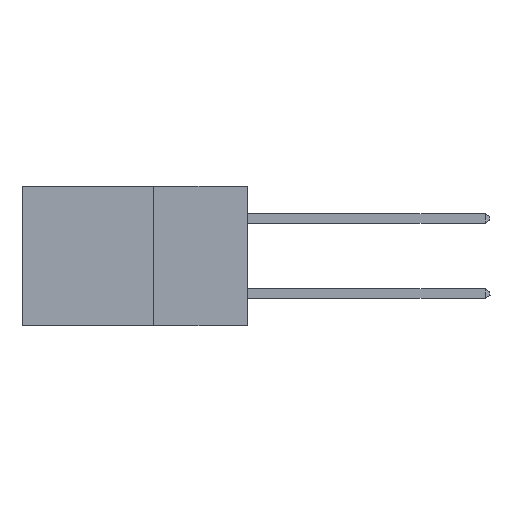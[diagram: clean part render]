
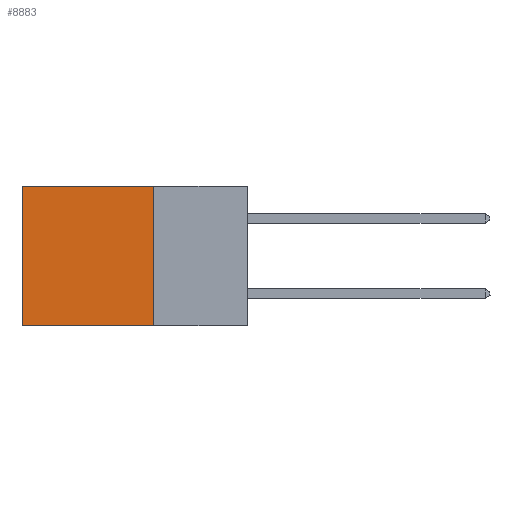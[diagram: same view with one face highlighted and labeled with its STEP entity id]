
A CAD part, left-side view. The second image highlights one B-rep face of the part: STEP entity #8883.
In plain terms, the highlighted planar face has unit normal (-1, 0, 0).
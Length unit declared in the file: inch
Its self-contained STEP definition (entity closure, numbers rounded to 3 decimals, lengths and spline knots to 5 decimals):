
#1209 = DIRECTION ( 'NONE',  ( 0., 0., -1. ) ) ;
#1258 = CARTESIAN_POINT ( 'NONE',  ( 0.298, 0.6, 0. ) ) ;
#1451 = CARTESIAN_POINT ( 'NONE',  ( 0.298, 0.6, 0. ) ) ;
#2287 = AXIS2_PLACEMENT_3D ( 'NONE', #20778, #7983, #25866 ) ;
#2558 = DIRECTION ( 'NONE',  ( 0., 1., 0. ) ) ;
#2759 = EDGE_CURVE ( 'NONE', #10760, #15663, #7163, .T. ) ;
#2866 = PLANE ( 'NONE',  #2287 ) ;
#3177 = EDGE_CURVE ( 'NONE', #23032, #15663, #19971, .T. ) ;
#6310 = VECTOR ( 'NONE', #15525, 39.37008 ) ;
#6875 = EDGE_CURVE ( 'NONE', #24932, #23032, #23200, .T. ) ;
#7163 = LINE ( 'NONE', #24477, #32726 ) ;
#7983 = DIRECTION ( 'NONE',  ( 1., 0., 0. ) ) ;
#8221 = EDGE_CURVE ( 'NONE', #24932, #10760, #19935, .T. ) ;
#8757 = VECTOR ( 'NONE', #2558, 39.37008 ) ;
#8883 = ADVANCED_FACE ( 'NONE', ( #32237 ), #2866, .F. ) ;
#10760 = VERTEX_POINT ( 'NONE', #13992 ) ;
#13992 = CARTESIAN_POINT ( 'NONE',  ( 0.298, 0.25, -0.37 ) ) ;
#15293 = CARTESIAN_POINT ( 'NONE',  ( 0.298, 0.25, 0. ) ) ;
#15525 = DIRECTION ( 'NONE',  ( 0., 0., -1. ) ) ;
#15663 = VERTEX_POINT ( 'NONE', #16317 ) ;
#16317 = CARTESIAN_POINT ( 'NONE',  ( 0.298, 0.6, -0.37 ) ) ;
#18099 = ORIENTED_EDGE ( 'NONE', *, *, #6875, .T. ) ;
#19935 = LINE ( 'NONE', #25678, #6310 ) ;
#19971 = LINE ( 'NONE', #1451, #32699 ) ;
#20778 = CARTESIAN_POINT ( 'NONE',  ( 0.298, 0.25, 0. ) ) ;
#21219 = CARTESIAN_POINT ( 'NONE',  ( 0.298, 0.25, 0. ) ) ;
#23032 = VERTEX_POINT ( 'NONE', #1258 ) ;
#23200 = LINE ( 'NONE', #15293, #8757 ) ;
#23925 = DIRECTION ( 'NONE',  ( 0., 1., 0. ) ) ;
#24385 = ORIENTED_EDGE ( 'NONE', *, *, #8221, .F. ) ;
#24477 = CARTESIAN_POINT ( 'NONE',  ( 0.298, 0.25, -0.37 ) ) ;
#24932 = VERTEX_POINT ( 'NONE', #21219 ) ;
#25008 = ORIENTED_EDGE ( 'NONE', *, *, #3177, .T. ) ;
#25678 = CARTESIAN_POINT ( 'NONE',  ( 0.298, 0.25, 0. ) ) ;
#25866 = DIRECTION ( 'NONE',  ( 0., 0., -1. ) ) ;
#28529 = ORIENTED_EDGE ( 'NONE', *, *, #2759, .F. ) ;
#30183 = EDGE_LOOP ( 'NONE', ( #25008, #28529, #24385, #18099 ) ) ;
#32237 = FACE_OUTER_BOUND ( 'NONE', #30183, .T. ) ;
#32699 = VECTOR ( 'NONE', #1209, 39.37008 ) ;
#32726 = VECTOR ( 'NONE', #23925, 39.37008 ) ;
